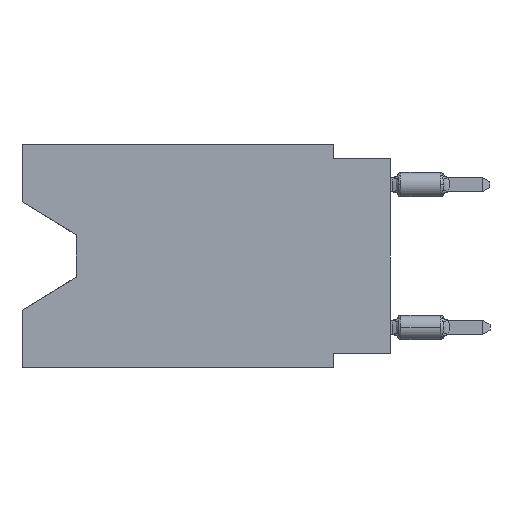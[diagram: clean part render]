
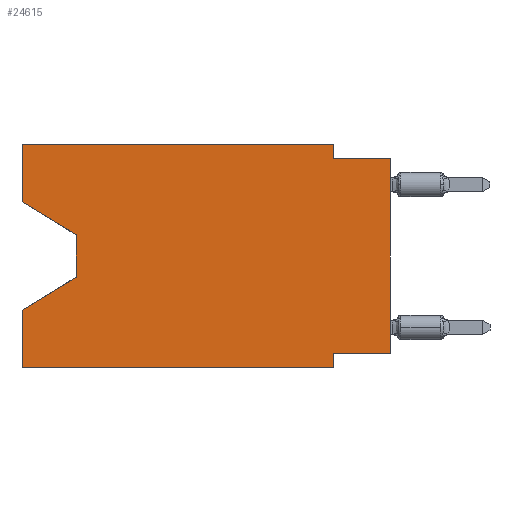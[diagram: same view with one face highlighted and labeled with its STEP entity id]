
A CAD part, left-side view. The second image highlights one B-rep face of the part: STEP entity #24615.
In plain terms, the highlighted planar face has unit normal (-1, 0, 0).
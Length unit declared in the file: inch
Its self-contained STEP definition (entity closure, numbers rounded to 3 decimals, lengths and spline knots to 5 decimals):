
#157 = VERTEX_POINT ( 'NONE', #52074 ) ;
#364 = ORIENTED_EDGE ( 'NONE', *, *, #32607, .F. ) ;
#407 = EDGE_CURVE ( 'NONE', #16330, #157, #2226, .T. ) ;
#783 = LINE ( 'NONE', #4669, #15334 ) ;
#1413 = VERTEX_POINT ( 'NONE', #45494 ) ;
#1939 = CARTESIAN_POINT ( 'NONE',  ( 0., 0.645, -0.10025 ) ) ;
#2210 = EDGE_CURVE ( 'NONE', #21622, #16330, #25742, .T. ) ;
#2226 = LINE ( 'NONE', #19231, #28875 ) ;
#2292 = DIRECTION ( 'NONE',  ( 0., -1., 0. ) ) ;
#3201 = LINE ( 'NONE', #15203, #11899 ) ;
#3991 = VERTEX_POINT ( 'NONE', #54061 ) ;
#4669 = CARTESIAN_POINT ( 'NONE',  ( 0., 0.645, -0.39 ) ) ;
#4707 = EDGE_CURVE ( 'NONE', #1413, #157, #783, .T. ) ;
#5111 = ORIENTED_EDGE ( 'NONE', *, *, #12660, .T. ) ;
#5197 = DIRECTION ( 'NONE',  ( 1., 0., 0. ) ) ;
#5215 = DIRECTION ( 'NONE',  ( 0., -1., 0. ) ) ;
#6856 = VECTOR ( 'NONE', #30110, 39.37008 ) ;
#7699 = VERTEX_POINT ( 'NONE', #54276 ) ;
#10246 = FACE_OUTER_BOUND ( 'NONE', #48933, .T. ) ;
#10404 = ORIENTED_EDGE ( 'NONE', *, *, #4707, .T. ) ;
#10506 = EDGE_CURVE ( 'NONE', #7699, #39877, #35210, .T. ) ;
#10595 = LINE ( 'NONE', #1939, #39311 ) ;
#11155 = CARTESIAN_POINT ( 'NONE',  ( 0., 0.645, -0.28975 ) ) ;
#11205 = LINE ( 'NONE', #24803, #48035 ) ;
#11899 = VECTOR ( 'NONE', #20204, 39.37008 ) ;
#12278 = CARTESIAN_POINT ( 'NONE',  ( 0., 0., -0.365 ) ) ;
#12308 = ORIENTED_EDGE ( 'NONE', *, *, #41582, .T. ) ;
#12660 = EDGE_CURVE ( 'NONE', #7699, #24671, #10595, .T. ) ;
#13170 = ORIENTED_EDGE ( 'NONE', *, *, #20184, .T. ) ;
#13583 = CARTESIAN_POINT ( 'NONE',  ( 0., 0.645, 0. ) ) ;
#13889 = EDGE_CURVE ( 'NONE', #3991, #40389, #21815, .T. ) ;
#15203 = CARTESIAN_POINT ( 'NONE',  ( 0., 0.645, 0. ) ) ;
#15274 = ORIENTED_EDGE ( 'NONE', *, *, #407, .F. ) ;
#15334 = VECTOR ( 'NONE', #5215, 39.37008 ) ;
#16330 = VERTEX_POINT ( 'NONE', #34396 ) ;
#16396 = ORIENTED_EDGE ( 'NONE', *, *, #44807, .F. ) ;
#17044 = CARTESIAN_POINT ( 'NONE',  ( 0., 0.55, -0.232 ) ) ;
#17190 = VECTOR ( 'NONE', #44459, 39.37008 ) ;
#17662 = DIRECTION ( 'NONE',  ( 0., 1., 0. ) ) ;
#18519 = ORIENTED_EDGE ( 'NONE', *, *, #50142, .T. ) ;
#18577 = CARTESIAN_POINT ( 'NONE',  ( 0., 0.1, 0. ) ) ;
#19231 = CARTESIAN_POINT ( 'NONE',  ( 0., 0.1, -0.39 ) ) ;
#20184 = EDGE_CURVE ( 'NONE', #48214, #54108, #38214, .T. ) ;
#20204 = DIRECTION ( 'NONE',  ( 0., 0., 1. ) ) ;
#20687 = VECTOR ( 'NONE', #31171, 39.37008 ) ;
#21244 = CARTESIAN_POINT ( 'NONE',  ( 0., 0., -0.025 ) ) ;
#21270 = VECTOR ( 'NONE', #21572, 39.37008 ) ;
#21572 = DIRECTION ( 'NONE',  ( 0., 0., 1. ) ) ;
#21622 = VERTEX_POINT ( 'NONE', #12278 ) ;
#21815 = LINE ( 'NONE', #21244, #25158 ) ;
#22829 = LINE ( 'NONE', #23099, #20687 ) ;
#23099 = CARTESIAN_POINT ( 'NONE',  ( 0., 0., 0. ) ) ;
#23396 = DIRECTION ( 'NONE',  ( 0., -0.855, -0.519 ) ) ;
#23804 = ORIENTED_EDGE ( 'NONE', *, *, #13889, .F. ) ;
#24615 = ADVANCED_FACE ( 'NONE', ( #10246 ), #43627, .F. ) ;
#24671 = VERTEX_POINT ( 'NONE', #48079 ) ;
#24803 = CARTESIAN_POINT ( 'NONE',  ( 0., 0.645, 0. ) ) ;
#25158 = VECTOR ( 'NONE', #51577, 39.37008 ) ;
#25742 = LINE ( 'NONE', #34641, #26030 ) ;
#25924 = VERTEX_POINT ( 'NONE', #42233 ) ;
#26030 = VECTOR ( 'NONE', #17662, 39.37008 ) ;
#28875 = VECTOR ( 'NONE', #36193, 39.37008 ) ;
#29574 = EDGE_CURVE ( 'NONE', #39877, #25924, #11205, .T. ) ;
#30110 = DIRECTION ( 'NONE',  ( 0., 0., -1. ) ) ;
#30184 = CARTESIAN_POINT ( 'NONE',  ( 0., 0.55, -0.232 ) ) ;
#30385 = LINE ( 'NONE', #50973, #6856 ) ;
#30569 = DIRECTION ( 'NONE',  ( 0., 0., -1. ) ) ;
#31171 = DIRECTION ( 'NONE',  ( 0., 0., 1. ) ) ;
#32607 = EDGE_CURVE ( 'NONE', #25924, #3991, #39726, .T. ) ;
#32998 = ORIENTED_EDGE ( 'NONE', *, *, #2210, .F. ) ;
#34314 = DIRECTION ( 'NONE',  ( 0., 0.855, -0.519 ) ) ;
#34396 = CARTESIAN_POINT ( 'NONE',  ( 0., 0.1, -0.365 ) ) ;
#34641 = CARTESIAN_POINT ( 'NONE',  ( 0., 0., -0.365 ) ) ;
#35210 = LINE ( 'NONE', #38560, #21270 ) ;
#35454 = ORIENTED_EDGE ( 'NONE', *, *, #29574, .F. ) ;
#36193 = DIRECTION ( 'NONE',  ( 0., 0., -1. ) ) ;
#38214 = LINE ( 'NONE', #17044, #40146 ) ;
#38560 = CARTESIAN_POINT ( 'NONE',  ( 0., 0.645, 0. ) ) ;
#39311 = VECTOR ( 'NONE', #23396, 39.37008 ) ;
#39726 = LINE ( 'NONE', #18577, #17190 ) ;
#39877 = VERTEX_POINT ( 'NONE', #47364 ) ;
#40146 = VECTOR ( 'NONE', #34314, 39.37008 ) ;
#40389 = VERTEX_POINT ( 'NONE', #48418 ) ;
#40851 = ORIENTED_EDGE ( 'NONE', *, *, #10506, .F. ) ;
#41582 = EDGE_CURVE ( 'NONE', #21622, #40389, #22829, .T. ) ;
#42233 = CARTESIAN_POINT ( 'NONE',  ( 0., 0.1, 0. ) ) ;
#43627 = PLANE ( 'NONE',  #50081 ) ;
#44459 = DIRECTION ( 'NONE',  ( 0., 0., -1. ) ) ;
#44807 = EDGE_CURVE ( 'NONE', #1413, #54108, #3201, .T. ) ;
#45494 = CARTESIAN_POINT ( 'NONE',  ( 0., 0.645, -0.39 ) ) ;
#47364 = CARTESIAN_POINT ( 'NONE',  ( 0., 0.645, 0. ) ) ;
#48035 = VECTOR ( 'NONE', #2292, 39.37008 ) ;
#48079 = CARTESIAN_POINT ( 'NONE',  ( 0., 0.55, -0.158 ) ) ;
#48214 = VERTEX_POINT ( 'NONE', #30184 ) ;
#48418 = CARTESIAN_POINT ( 'NONE',  ( 0., 0., -0.025 ) ) ;
#48933 = EDGE_LOOP ( 'NONE', ( #5111, #18519, #13170, #16396, #10404, #15274, #32998, #12308, #23804, #364, #35454, #40851 ) ) ;
#50081 = AXIS2_PLACEMENT_3D ( 'NONE', #13583, #5197, #30569 ) ;
#50142 = EDGE_CURVE ( 'NONE', #24671, #48214, #30385, .T. ) ;
#50973 = CARTESIAN_POINT ( 'NONE',  ( 0., 0.55, -0.158 ) ) ;
#51577 = DIRECTION ( 'NONE',  ( 0., -1., 0. ) ) ;
#52074 = CARTESIAN_POINT ( 'NONE',  ( 0., 0.1, -0.39 ) ) ;
#54061 = CARTESIAN_POINT ( 'NONE',  ( 0., 0.1, -0.025 ) ) ;
#54108 = VERTEX_POINT ( 'NONE', #11155 ) ;
#54276 = CARTESIAN_POINT ( 'NONE',  ( 0., 0.645, -0.10025 ) ) ;
